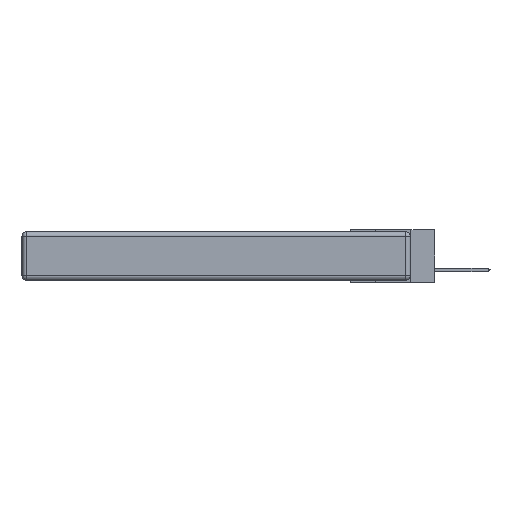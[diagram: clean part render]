
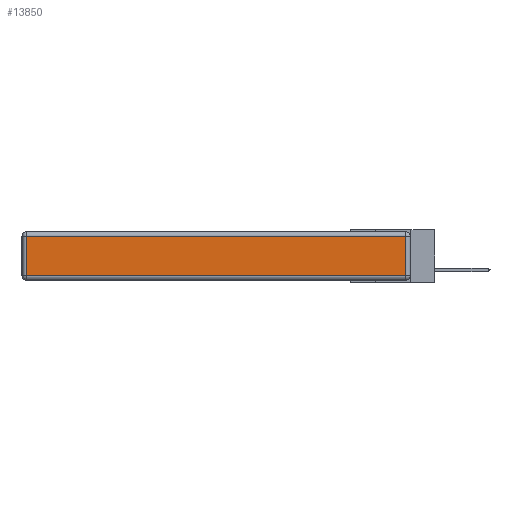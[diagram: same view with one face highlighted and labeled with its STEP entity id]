
A CAD part, left-side view. The second image highlights one B-rep face of the part: STEP entity #13850.
In plain terms, the highlighted planar face has unit normal (-1, 0, 0).
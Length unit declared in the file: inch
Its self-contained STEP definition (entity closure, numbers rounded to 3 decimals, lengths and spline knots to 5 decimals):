
#4 = EDGE_CURVE ( 'NONE', #1052, #2053, #3995, .T. ) ;
#724 = ORIENTED_EDGE ( 'NONE', *, *, #16462, .T. ) ;
#1052 = VERTEX_POINT ( 'NONE', #7913 ) ;
#1322 = CARTESIAN_POINT ( 'NONE',  ( 0., 0., -0.313 ) ) ;
#1717 = ORIENTED_EDGE ( 'NONE', *, *, #5569, .T. ) ;
#2053 = VERTEX_POINT ( 'NONE', #11824 ) ;
#2812 = EDGE_CURVE ( 'NONE', #5858, #12368, #16485, .T. ) ;
#3225 = ORIENTED_EDGE ( 'NONE', *, *, #2812, .T. ) ;
#3301 = CARTESIAN_POINT ( 'NONE',  ( 0., 0.03, -0.03 ) ) ;
#3801 = VECTOR ( 'NONE', #19522, 39.37008 ) ;
#3995 = LINE ( 'NONE', #20204, #12926 ) ;
#5569 = EDGE_CURVE ( 'NONE', #12368, #1052, #21401, .T. ) ;
#5721 = EDGE_LOOP ( 'NONE', ( #724, #3225, #1717, #12774 ) ) ;
#5858 = VERTEX_POINT ( 'NONE', #9075 ) ;
#7913 = CARTESIAN_POINT ( 'NONE',  ( 0., 2.72, -0.03 ) ) ;
#7930 = DIRECTION ( 'NONE',  ( -1., 0., 0. ) ) ;
#9075 = CARTESIAN_POINT ( 'NONE',  ( 0., 0.03, -0.313 ) ) ;
#9429 = CARTESIAN_POINT ( 'NONE',  ( 0., 2.75, -0.03 ) ) ;
#11824 = CARTESIAN_POINT ( 'NONE',  ( 0., 2.72, -0.313 ) ) ;
#12368 = VERTEX_POINT ( 'NONE', #3301 ) ;
#12690 = DIRECTION ( 'NONE',  ( 0., 0., 1. ) ) ;
#12774 = ORIENTED_EDGE ( 'NONE', *, *, #4, .T. ) ;
#12926 = VECTOR ( 'NONE', #15196, 39.37008 ) ;
#13389 = AXIS2_PLACEMENT_3D ( 'NONE', #14528, #7930, #21411 ) ;
#13850 = ADVANCED_FACE ( 'NONE', ( #17339 ), #16167, .T. ) ;
#14169 = DIRECTION ( 'NONE',  ( 0., 1., 0. ) ) ;
#14517 = VECTOR ( 'NONE', #14169, 39.37008 ) ;
#14528 = CARTESIAN_POINT ( 'NONE',  ( 0., 0., -0.343 ) ) ;
#15196 = DIRECTION ( 'NONE',  ( 0., 0., -1. ) ) ;
#16167 = PLANE ( 'NONE',  #13389 ) ;
#16462 = EDGE_CURVE ( 'NONE', #2053, #5858, #17221, .T. ) ;
#16485 = LINE ( 'NONE', #17661, #17845 ) ;
#17221 = LINE ( 'NONE', #1322, #3801 ) ;
#17339 = FACE_OUTER_BOUND ( 'NONE', #5721, .T. ) ;
#17661 = CARTESIAN_POINT ( 'NONE',  ( 0., 0.03, -0.343 ) ) ;
#17845 = VECTOR ( 'NONE', #12690, 39.37008 ) ;
#19522 = DIRECTION ( 'NONE',  ( 0., -1., 0. ) ) ;
#20204 = CARTESIAN_POINT ( 'NONE',  ( 0., 2.72, -0.343 ) ) ;
#21401 = LINE ( 'NONE', #9429, #14517 ) ;
#21411 = DIRECTION ( 'NONE',  ( 0., 0., 1. ) ) ;
